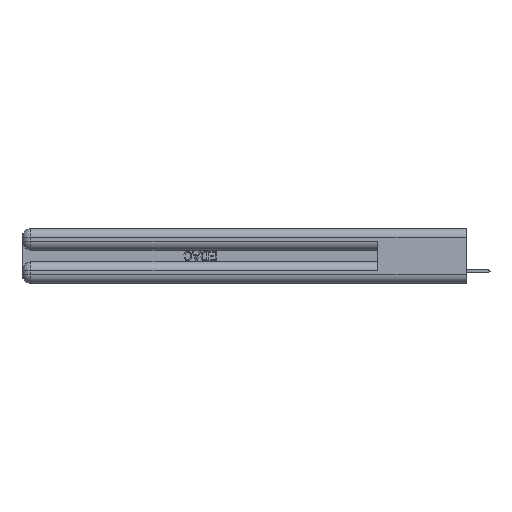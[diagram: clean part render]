
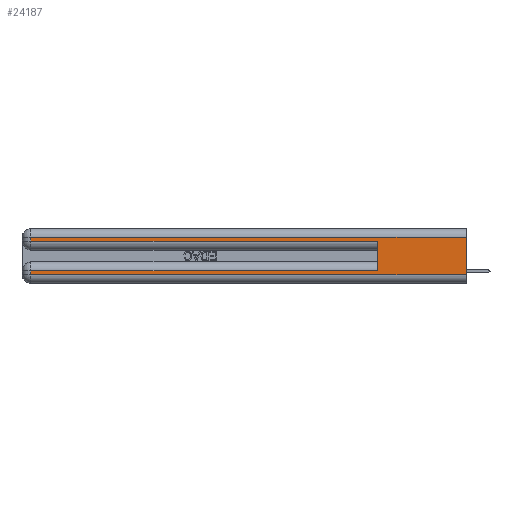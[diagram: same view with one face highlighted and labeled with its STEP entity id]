
A CAD part, left-side view. The second image highlights one B-rep face of the part: STEP entity #24187.
In plain terms, the highlighted planar face has unit normal (-1, 0, 0).
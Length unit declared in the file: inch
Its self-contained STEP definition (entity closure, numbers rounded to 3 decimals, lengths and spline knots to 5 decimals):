
#2334 = ORIENTED_EDGE ( 'NONE', *, *, #48511, .T. ) ;
#3852 = VERTEX_POINT ( 'NONE', #13879 ) ;
#4071 = VERTEX_POINT ( 'NONE', #10333 ) ;
#5620 = CARTESIAN_POINT ( 'NONE',  ( 0., 0., 0.06 ) ) ;
#7026 = CARTESIAN_POINT ( 'NONE',  ( 0., 0., 0.085 ) ) ;
#7384 = DIRECTION ( 'NONE',  ( 0., 0., -1. ) ) ;
#8671 = EDGE_LOOP ( 'NONE', ( #31113, #27071, #21857, #2334, #41377, #39354, #31205, #17270 ) ) ;
#8797 = DIRECTION ( 'NONE',  ( 0., -1., 0. ) ) ;
#8987 = VECTOR ( 'NONE', #28610, 39.37008 ) ;
#10333 = CARTESIAN_POINT ( 'NONE',  ( 0., 0., 0.31 ) ) ;
#11583 = DIRECTION ( 'NONE',  ( 0., 0., -1. ) ) ;
#11645 = DIRECTION ( 'NONE',  ( 1., 0., 0. ) ) ;
#13879 = CARTESIAN_POINT ( 'NONE',  ( 0., 2.94, 0.285 ) ) ;
#14482 = VERTEX_POINT ( 'NONE', #48873 ) ;
#14600 = FACE_OUTER_BOUND ( 'NONE', #8671, .T. ) ;
#14669 = DIRECTION ( 'NONE',  ( 0., 0., -1. ) ) ;
#15265 = CARTESIAN_POINT ( 'NONE',  ( 0., 0., 0.06 ) ) ;
#15353 = PLANE ( 'NONE',  #46399 ) ;
#15374 = DIRECTION ( 'NONE',  ( 0., 0., -1. ) ) ;
#16854 = CARTESIAN_POINT ( 'NONE',  ( 0., 2.94, 0.085 ) ) ;
#16933 = VERTEX_POINT ( 'NONE', #51268 ) ;
#17270 = ORIENTED_EDGE ( 'NONE', *, *, #32641, .T. ) ;
#18555 = CARTESIAN_POINT ( 'NONE',  ( 0., 2.94, 0.37 ) ) ;
#18617 = CARTESIAN_POINT ( 'NONE',  ( 0., 0.6, 0.085 ) ) ;
#19285 = EDGE_CURVE ( 'NONE', #16933, #3852, #35408, .T. ) ;
#20278 = LINE ( 'NONE', #50396, #40850 ) ;
#21857 = ORIENTED_EDGE ( 'NONE', *, *, #19285, .T. ) ;
#21934 = LINE ( 'NONE', #44316, #35541 ) ;
#23551 = VECTOR ( 'NONE', #26151, 39.37008 ) ;
#23968 = CARTESIAN_POINT ( 'NONE',  ( 0., 0., 0.37 ) ) ;
#24187 = ADVANCED_FACE ( 'NONE', ( #14600 ), #15353, .F. ) ;
#25661 = VERTEX_POINT ( 'NONE', #18617 ) ;
#25686 = VERTEX_POINT ( 'NONE', #15265 ) ;
#25863 = EDGE_CURVE ( 'NONE', #25661, #45144, #44527, .T. ) ;
#26151 = DIRECTION ( 'NONE',  ( 0., -1., 0. ) ) ;
#26161 = EDGE_CURVE ( 'NONE', #45144, #14482, #21934, .T. ) ;
#27071 = ORIENTED_EDGE ( 'NONE', *, *, #41280, .T. ) ;
#27151 = CARTESIAN_POINT ( 'NONE',  ( 0., 0., 0.285 ) ) ;
#28610 = DIRECTION ( 'NONE',  ( 0., 0., 1. ) ) ;
#28880 = LINE ( 'NONE', #48995, #8987 ) ;
#31113 = ORIENTED_EDGE ( 'NONE', *, *, #31705, .F. ) ;
#31205 = ORIENTED_EDGE ( 'NONE', *, *, #26161, .T. ) ;
#31681 = CARTESIAN_POINT ( 'NONE',  ( 0., 0.6, 0.285 ) ) ;
#31705 = EDGE_CURVE ( 'NONE', #4071, #25686, #46622, .T. ) ;
#32641 = EDGE_CURVE ( 'NONE', #14482, #25686, #37601, .T. ) ;
#33847 = VECTOR ( 'NONE', #15374, 39.37008 ) ;
#34345 = DIRECTION ( 'NONE',  ( 0., 1., 0. ) ) ;
#35408 = LINE ( 'NONE', #18555, #36104 ) ;
#35541 = VECTOR ( 'NONE', #11583, 39.37008 ) ;
#36104 = VECTOR ( 'NONE', #14669, 39.37008 ) ;
#36173 = EDGE_CURVE ( 'NONE', #25661, #38134, #28880, .T. ) ;
#37601 = LINE ( 'NONE', #5620, #23551 ) ;
#38134 = VERTEX_POINT ( 'NONE', #31681 ) ;
#39354 = ORIENTED_EDGE ( 'NONE', *, *, #25863, .T. ) ;
#39404 = VECTOR ( 'NONE', #40275, 39.37008 ) ;
#39534 = VECTOR ( 'NONE', #8797, 39.37008 ) ;
#40275 = DIRECTION ( 'NONE',  ( 0., 1., 0. ) ) ;
#40850 = VECTOR ( 'NONE', #34345, 39.37008 ) ;
#41280 = EDGE_CURVE ( 'NONE', #4071, #16933, #20278, .T. ) ;
#41377 = ORIENTED_EDGE ( 'NONE', *, *, #36173, .F. ) ;
#44316 = CARTESIAN_POINT ( 'NONE',  ( 0., 2.94, 0.37 ) ) ;
#44527 = LINE ( 'NONE', #7026, #39404 ) ;
#45144 = VERTEX_POINT ( 'NONE', #16854 ) ;
#46399 = AXIS2_PLACEMENT_3D ( 'NONE', #47970, #11645, #7384 ) ;
#46622 = LINE ( 'NONE', #23968, #33847 ) ;
#47970 = CARTESIAN_POINT ( 'NONE',  ( 0., 0., 0.37 ) ) ;
#48511 = EDGE_CURVE ( 'NONE', #3852, #38134, #51684, .T. ) ;
#48873 = CARTESIAN_POINT ( 'NONE',  ( 0., 2.94, 0.06 ) ) ;
#48995 = CARTESIAN_POINT ( 'NONE',  ( 0., 0.6, 0.145 ) ) ;
#50396 = CARTESIAN_POINT ( 'NONE',  ( 0., 0., 0.31 ) ) ;
#51268 = CARTESIAN_POINT ( 'NONE',  ( 0., 2.94, 0.31 ) ) ;
#51684 = LINE ( 'NONE', #27151, #39534 ) ;
